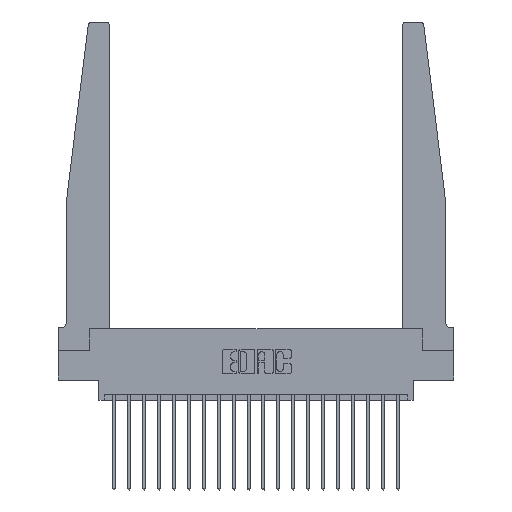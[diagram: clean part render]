
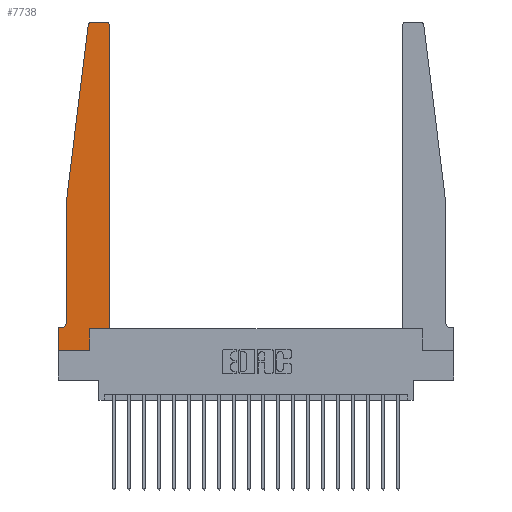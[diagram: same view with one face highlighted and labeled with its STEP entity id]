
A CAD part, top view. The second image highlights one B-rep face of the part: STEP entity #7738.
In plain terms, the highlighted planar face has unit normal (0, 0, 1).
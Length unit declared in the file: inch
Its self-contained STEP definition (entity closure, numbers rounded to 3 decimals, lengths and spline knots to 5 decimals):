
#89 = DIRECTION ( 'NONE',  ( 1., 0., 0. ) ) ;
#158 = DIRECTION ( 'NONE',  ( 1., 0., 0. ) ) ;
#185 = CARTESIAN_POINT ( 'NONE',  ( 0.065, 0.2375, 0.37 ) ) ;
#297 = VERTEX_POINT ( 'NONE', #7095 ) ;
#659 = DIRECTION ( 'NONE',  ( 0., -1., 0. ) ) ;
#679 = VECTOR ( 'NONE', #158, 39.37008 ) ;
#1187 = LINE ( 'NONE', #11512, #679 ) ;
#1719 = VERTEX_POINT ( 'NONE', #6671 ) ;
#1794 = ORIENTED_EDGE ( 'NONE', *, *, #17437, .T. ) ;
#1801 = CARTESIAN_POINT ( 'NONE',  ( 0.24675, 2.72367, 0.37 ) ) ;
#1812 = ORIENTED_EDGE ( 'NONE', *, *, #11732, .T. ) ;
#1974 = VERTEX_POINT ( 'NONE', #3588 ) ;
#2122 = CARTESIAN_POINT ( 'NONE',  ( 0.065, 1.25, 0.37 ) ) ;
#2347 = EDGE_CURVE ( 'NONE', #12516, #12687, #19662, .T. ) ;
#2796 = DIRECTION ( 'NONE',  ( 0., 0., 1. ) ) ;
#2836 = CARTESIAN_POINT ( 'NONE',  ( 0., 0., 0.37 ) ) ;
#2986 = VECTOR ( 'NONE', #89, 39.37008 ) ;
#3074 = LINE ( 'NONE', #5510, #19751 ) ;
#3090 = EDGE_CURVE ( 'NONE', #13349, #297, #3735, .T. ) ;
#3588 = CARTESIAN_POINT ( 'NONE',  ( 0.425, 2.72, 0.37 ) ) ;
#3713 = ORIENTED_EDGE ( 'NONE', *, *, #2347, .T. ) ;
#3732 = EDGE_CURVE ( 'NONE', #6293, #12516, #10287, .T. ) ;
#3735 = LINE ( 'NONE', #16758, #16091 ) ;
#4371 = FACE_OUTER_BOUND ( 'NONE', #18093, .T. ) ;
#4663 = AXIS2_PLACEMENT_3D ( 'NONE', #12461, #2796, #14086 ) ;
#4882 = VECTOR ( 'NONE', #8584, 39.37008 ) ;
#5148 = DIRECTION ( 'NONE',  ( 0., 0., -1. ) ) ;
#5431 = CARTESIAN_POINT ( 'NONE',  ( 0.395, 2.75, 0.37 ) ) ;
#5461 = LINE ( 'NONE', #2122, #18348 ) ;
#5510 = CARTESIAN_POINT ( 'NONE',  ( 0., 0., 0.37 ) ) ;
#5617 = VECTOR ( 'NONE', #19989, 39.37008 ) ;
#5708 = DIRECTION ( 'NONE',  ( 0., -1., 0. ) ) ;
#5815 = ORIENTED_EDGE ( 'NONE', *, *, #13179, .T. ) ;
#6131 = LINE ( 'NONE', #11943, #5617 ) ;
#6172 = EDGE_CURVE ( 'NONE', #1974, #13349, #19006, .T. ) ;
#6293 = VERTEX_POINT ( 'NONE', #15924 ) ;
#6574 = EDGE_CURVE ( 'NONE', #11607, #1974, #8686, .T. ) ;
#6671 = CARTESIAN_POINT ( 'NONE',  ( 0.2605, 0.18, 0.37 ) ) ;
#6775 = DIRECTION ( 'NONE',  ( 0., 0., 1. ) ) ;
#6938 = CARTESIAN_POINT ( 'NONE',  ( 0.27653, 2.72, 0.37 ) ) ;
#6959 = CARTESIAN_POINT ( 'NONE',  ( 0.425, 0.18, 0.37 ) ) ;
#6985 = LINE ( 'NONE', #20168, #18847 ) ;
#7095 = CARTESIAN_POINT ( 'NONE',  ( 0.27653, 2.75, 0.37 ) ) ;
#7571 = ORIENTED_EDGE ( 'NONE', *, *, #3090, .T. ) ;
#7687 = VERTEX_POINT ( 'NONE', #16284 ) ;
#7738 = ADVANCED_FACE ( 'NONE', ( #4371 ), #16426, .T. ) ;
#7905 = EDGE_CURVE ( 'NONE', #7961, #1719, #6131, .T. ) ;
#7961 = VERTEX_POINT ( 'NONE', #15327 ) ;
#8555 = DIRECTION ( 'NONE',  ( 1., 0., 0. ) ) ;
#8584 = DIRECTION ( 'NONE',  ( 0., 1., 0. ) ) ;
#8686 = LINE ( 'NONE', #6959, #4882 ) ;
#9520 = ORIENTED_EDGE ( 'NONE', *, *, #3732, .T. ) ;
#9820 = CARTESIAN_POINT ( 'NONE',  ( 0., 0., 0.37 ) ) ;
#10164 = VERTEX_POINT ( 'NONE', #1801 ) ;
#10287 = LINE ( 'NONE', #12141, #17336 ) ;
#11512 = CARTESIAN_POINT ( 'NONE',  ( 0.425, 0.18, 0.37 ) ) ;
#11607 = VERTEX_POINT ( 'NONE', #15028 ) ;
#11732 = EDGE_CURVE ( 'NONE', #12687, #7687, #6985, .T. ) ;
#11737 = AXIS2_PLACEMENT_3D ( 'NONE', #13181, #6775, #18062 ) ;
#11943 = CARTESIAN_POINT ( 'NONE',  ( 0.2605, 0.18, 0.37 ) ) ;
#12141 = CARTESIAN_POINT ( 'NONE',  ( 0.065, 1.25, 0.37 ) ) ;
#12332 = AXIS2_PLACEMENT_3D ( 'NONE', #14797, #5148, #16425 ) ;
#12334 = ORIENTED_EDGE ( 'NONE', *, *, #19216, .T. ) ;
#12461 = CARTESIAN_POINT ( 'NONE',  ( 0.395, 2.72, 0.37 ) ) ;
#12516 = VERTEX_POINT ( 'NONE', #185 ) ;
#12687 = VERTEX_POINT ( 'NONE', #16682 ) ;
#13179 = EDGE_CURVE ( 'NONE', #16954, #7961, #19658, .T. ) ;
#13181 = CARTESIAN_POINT ( 'NONE',  ( 0., 0.1875, 0.37 ) ) ;
#13330 = ORIENTED_EDGE ( 'NONE', *, *, #6172, .T. ) ;
#13349 = VERTEX_POINT ( 'NONE', #5431 ) ;
#13993 = ORIENTED_EDGE ( 'NONE', *, *, #20474, .T. ) ;
#14086 = DIRECTION ( 'NONE',  ( 1., 0., 0. ) ) ;
#14192 = CIRCLE ( 'NONE', #16723, 0.03 ) ;
#14783 = ORIENTED_EDGE ( 'NONE', *, *, #7905, .T. ) ;
#14797 = CARTESIAN_POINT ( 'NONE',  ( 0.015, 0.2375, 0.37 ) ) ;
#15028 = CARTESIAN_POINT ( 'NONE',  ( 0.425, 0.18, 0.37 ) ) ;
#15053 = DIRECTION ( 'NONE',  ( -0.122, -0.992, 0. ) ) ;
#15208 = DIRECTION ( 'NONE',  ( -1., 0., 0. ) ) ;
#15327 = CARTESIAN_POINT ( 'NONE',  ( 0.2605, 0., 0.37 ) ) ;
#15924 = CARTESIAN_POINT ( 'NONE',  ( 0.065, 1.25, 0.37 ) ) ;
#16091 = VECTOR ( 'NONE', #15208, 39.37008 ) ;
#16284 = CARTESIAN_POINT ( 'NONE',  ( 0., 0.1875, 0.37 ) ) ;
#16425 = DIRECTION ( 'NONE',  ( -1., 0., 0. ) ) ;
#16426 = PLANE ( 'NONE',  #11737 ) ;
#16682 = CARTESIAN_POINT ( 'NONE',  ( 0.015, 0.1875, 0.37 ) ) ;
#16723 = AXIS2_PLACEMENT_3D ( 'NONE', #6938, #18228, #8555 ) ;
#16758 = CARTESIAN_POINT ( 'NONE',  ( 0.25, 2.75, 0.37 ) ) ;
#16954 = VERTEX_POINT ( 'NONE', #2836 ) ;
#16999 = DIRECTION ( 'NONE',  ( -1., 0., 0. ) ) ;
#17262 = ORIENTED_EDGE ( 'NONE', *, *, #17354, .T. ) ;
#17336 = VECTOR ( 'NONE', #5708, 39.37008 ) ;
#17354 = EDGE_CURVE ( 'NONE', #297, #10164, #14192, .T. ) ;
#17437 = EDGE_CURVE ( 'NONE', #7687, #16954, #3074, .T. ) ;
#18062 = DIRECTION ( 'NONE',  ( 1., 0., 0. ) ) ;
#18093 = EDGE_LOOP ( 'NONE', ( #7571, #17262, #13993, #9520, #3713, #1812, #1794, #5815, #14783, #12334, #18317, #13330 ) ) ;
#18228 = DIRECTION ( 'NONE',  ( 0., 0., 1. ) ) ;
#18317 = ORIENTED_EDGE ( 'NONE', *, *, #6574, .T. ) ;
#18348 = VECTOR ( 'NONE', #15053, 39.37008 ) ;
#18847 = VECTOR ( 'NONE', #16999, 39.37008 ) ;
#19006 = CIRCLE ( 'NONE', #4663, 0.03 ) ;
#19216 = EDGE_CURVE ( 'NONE', #1719, #11607, #1187, .T. ) ;
#19658 = LINE ( 'NONE', #9820, #2986 ) ;
#19662 = CIRCLE ( 'NONE', #12332, 0.05 ) ;
#19751 = VECTOR ( 'NONE', #659, 39.37008 ) ;
#19989 = DIRECTION ( 'NONE',  ( 0., 1., 0. ) ) ;
#20168 = CARTESIAN_POINT ( 'NONE',  ( 0.065, 0.1875, 0.37 ) ) ;
#20474 = EDGE_CURVE ( 'NONE', #10164, #6293, #5461, .T. ) ;
